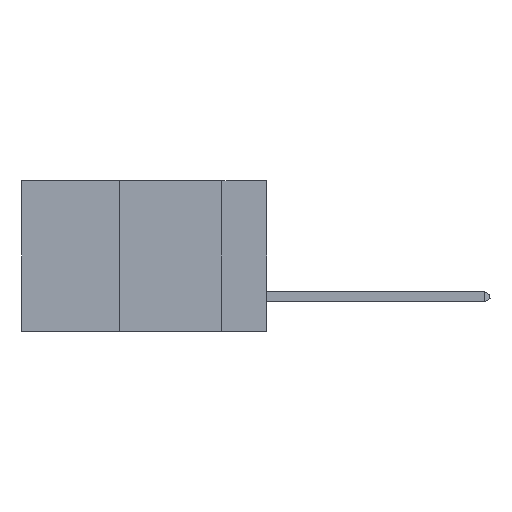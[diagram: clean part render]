
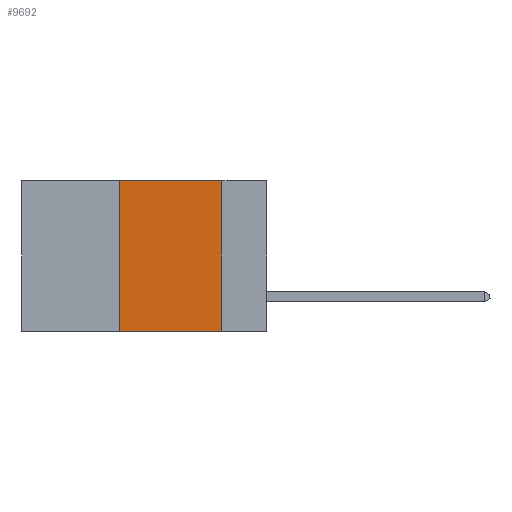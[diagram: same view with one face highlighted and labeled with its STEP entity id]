
A CAD part, left-side view. The second image highlights one B-rep face of the part: STEP entity #9692.
In plain terms, the highlighted planar face has unit normal (-1, 0, 0).
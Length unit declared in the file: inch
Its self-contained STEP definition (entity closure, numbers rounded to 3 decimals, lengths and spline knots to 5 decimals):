
#1417 = CARTESIAN_POINT ( 'NONE',  ( 0., 0.36, 0. ) ) ;
#2894 = ORIENTED_EDGE ( 'NONE', *, *, #19770, .F. ) ;
#3101 = DIRECTION ( 'NONE',  ( 0., -1., 0. ) ) ;
#5071 = CARTESIAN_POINT ( 'NONE',  ( 0., 0.11, -0.37 ) ) ;
#5792 = FACE_OUTER_BOUND ( 'NONE', #21467, .T. ) ;
#6606 = VECTOR ( 'NONE', #18056, 39.37008 ) ;
#6871 = DIRECTION ( 'NONE',  ( 0., 0., -1. ) ) ;
#9692 = ADVANCED_FACE ( 'NONE', ( #5792 ), #33899, .F. ) ;
#10864 = CARTESIAN_POINT ( 'NONE',  ( 0., 0.11, 0. ) ) ;
#11225 = VERTEX_POINT ( 'NONE', #33731 ) ;
#12409 = DIRECTION ( 'NONE',  ( 0., -1., 0. ) ) ;
#13254 = ORIENTED_EDGE ( 'NONE', *, *, #22898, .T. ) ;
#13423 = LINE ( 'NONE', #19871, #18621 ) ;
#16036 = AXIS2_PLACEMENT_3D ( 'NONE', #26027, #17666, #6871 ) ;
#17666 = DIRECTION ( 'NONE',  ( 1., 0., 0. ) ) ;
#17832 = CARTESIAN_POINT ( 'NONE',  ( 0., 0.6, 0. ) ) ;
#18056 = DIRECTION ( 'NONE',  ( 0., 0., -1. ) ) ;
#18618 = CARTESIAN_POINT ( 'NONE',  ( 0., 0.36, 0. ) ) ;
#18621 = VECTOR ( 'NONE', #3101, 39.37008 ) ;
#19770 = EDGE_CURVE ( 'NONE', #28185, #23309, #20594, .T. ) ;
#19871 = CARTESIAN_POINT ( 'NONE',  ( 0., 0.6, -0.37 ) ) ;
#20594 = LINE ( 'NONE', #17832, #33659 ) ;
#21136 = EDGE_CURVE ( 'NONE', #23309, #23743, #23179, .T. ) ;
#21467 = EDGE_LOOP ( 'NONE', ( #21816, #2894, #34005, #13254 ) ) ;
#21816 = ORIENTED_EDGE ( 'NONE', *, *, #21136, .F. ) ;
#22898 = EDGE_CURVE ( 'NONE', #11225, #23743, #13423, .T. ) ;
#23179 = LINE ( 'NONE', #23248, #6606 ) ;
#23248 = CARTESIAN_POINT ( 'NONE',  ( 0., 0.11, 0. ) ) ;
#23309 = VERTEX_POINT ( 'NONE', #10864 ) ;
#23743 = VERTEX_POINT ( 'NONE', #5071 ) ;
#24353 = LINE ( 'NONE', #18618, #30842 ) ;
#26027 = CARTESIAN_POINT ( 'NONE',  ( 0., 0.6, 0. ) ) ;
#28185 = VERTEX_POINT ( 'NONE', #1417 ) ;
#30842 = VECTOR ( 'NONE', #35292, 39.37008 ) ;
#31419 = EDGE_CURVE ( 'NONE', #11225, #28185, #24353, .T. ) ;
#33659 = VECTOR ( 'NONE', #12409, 39.37008 ) ;
#33731 = CARTESIAN_POINT ( 'NONE',  ( 0., 0.36, -0.37 ) ) ;
#33899 = PLANE ( 'NONE',  #16036 ) ;
#34005 = ORIENTED_EDGE ( 'NONE', *, *, #31419, .F. ) ;
#35292 = DIRECTION ( 'NONE',  ( 0., 0., 1. ) ) ;
